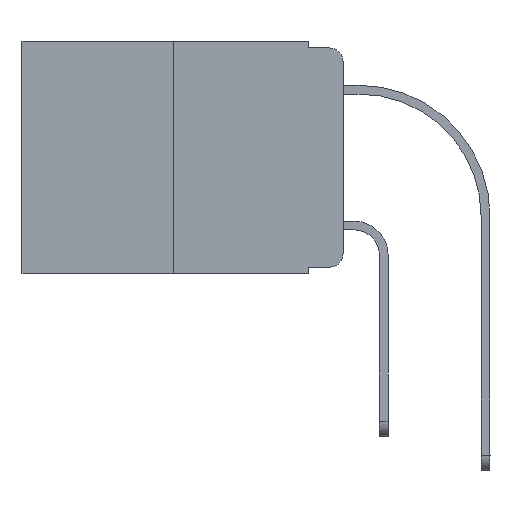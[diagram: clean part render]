
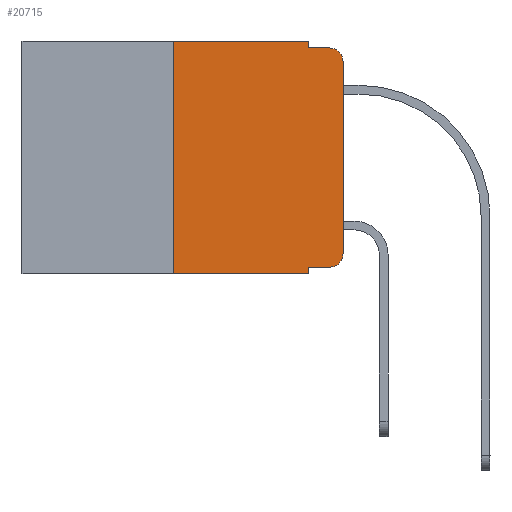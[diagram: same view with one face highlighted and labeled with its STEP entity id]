
A CAD part, left-side view. The second image highlights one B-rep face of the part: STEP entity #20715.
In plain terms, the highlighted planar face has unit normal (-1, 0, 0).
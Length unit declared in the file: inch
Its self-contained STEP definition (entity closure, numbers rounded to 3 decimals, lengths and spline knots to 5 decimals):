
#420 = DIRECTION ( 'NONE',  ( 0., 0., -1. ) ) ;
#704 = LINE ( 'NONE', #15815, #18201 ) ;
#1155 = CARTESIAN_POINT ( 'NONE',  ( 0., 0.051, -0.01 ) ) ;
#1318 = LINE ( 'NONE', #11101, #2013 ) ;
#1410 = EDGE_CURVE ( 'NONE', #24052, #24113, #2910, .T. ) ;
#1535 = DIRECTION ( 'NONE',  ( 0., -1., 0. ) ) ;
#2013 = VECTOR ( 'NONE', #20582, 39.37008 ) ;
#2109 = CARTESIAN_POINT ( 'NONE',  ( 0., 0.02, -0.01 ) ) ;
#2423 = EDGE_CURVE ( 'NONE', #16478, #14623, #15727, .T. ) ;
#2548 = ORIENTED_EDGE ( 'NONE', *, *, #1410, .F. ) ;
#2594 = LINE ( 'NONE', #12363, #2816 ) ;
#2816 = VECTOR ( 'NONE', #10336, 39.37008 ) ;
#2910 = LINE ( 'NONE', #12431, #20098 ) ;
#2971 = VERTEX_POINT ( 'NONE', #6167 ) ;
#3082 = ORIENTED_EDGE ( 'NONE', *, *, #23763, .T. ) ;
#3496 = VECTOR ( 'NONE', #12062, 39.37008 ) ;
#4196 = EDGE_CURVE ( 'NONE', #17796, #24052, #704, .T. ) ;
#4217 = LINE ( 'NONE', #7647, #15035 ) ;
#4219 = ORIENTED_EDGE ( 'NONE', *, *, #4196, .F. ) ;
#5891 = EDGE_CURVE ( 'NONE', #14530, #2971, #2594, .T. ) ;
#6167 = CARTESIAN_POINT ( 'NONE',  ( 0., 0., -0.03 ) ) ;
#7014 = CARTESIAN_POINT ( 'NONE',  ( 0., 0.473, 0. ) ) ;
#7241 = LINE ( 'NONE', #1155, #8109 ) ;
#7606 = ORIENTED_EDGE ( 'NONE', *, *, #24341, .T. ) ;
#7647 = CARTESIAN_POINT ( 'NONE',  ( 0., 0.051, 0. ) ) ;
#8109 = VECTOR ( 'NONE', #1535, 39.37008 ) ;
#8528 = CARTESIAN_POINT ( 'NONE',  ( 0., 0.051, 0. ) ) ;
#9140 = CARTESIAN_POINT ( 'NONE',  ( 0., 0.051, -0.01 ) ) ;
#9180 = DIRECTION ( 'NONE',  ( 0., 0., -1. ) ) ;
#9775 = VERTEX_POINT ( 'NONE', #9140 ) ;
#9787 = DIRECTION ( 'NONE',  ( 0., 0., -1. ) ) ;
#9946 = VECTOR ( 'NONE', #18331, 39.37008 ) ;
#10307 = VERTEX_POINT ( 'NONE', #2109 ) ;
#10336 = DIRECTION ( 'NONE',  ( 0., 0., 1. ) ) ;
#10537 = EDGE_CURVE ( 'NONE', #17796, #14623, #14666, .T. ) ;
#10985 = AXIS2_PLACEMENT_3D ( 'NONE', #15717, #17748, #9787 ) ;
#11101 = CARTESIAN_POINT ( 'NONE',  ( 0., 0.051, -0.333 ) ) ;
#11473 = DIRECTION ( 'NONE',  ( 0., 0., -1. ) ) ;
#11680 = VERTEX_POINT ( 'NONE', #16482 ) ;
#11714 = CARTESIAN_POINT ( 'NONE',  ( 0., 0., -0.313 ) ) ;
#11954 = CARTESIAN_POINT ( 'NONE',  ( 0., 0.051, -0.343 ) ) ;
#12062 = DIRECTION ( 'NONE',  ( 0., 0., -1. ) ) ;
#12363 = CARTESIAN_POINT ( 'NONE',  ( 0., 0., 0. ) ) ;
#12381 = CARTESIAN_POINT ( 'NONE',  ( 0., 0.473, -0.343 ) ) ;
#12431 = CARTESIAN_POINT ( 'NONE',  ( 0., 0.473, 0. ) ) ;
#13005 = DIRECTION ( 'NONE',  ( -1., 0., 0. ) ) ;
#13034 = ORIENTED_EDGE ( 'NONE', *, *, #2423, .F. ) ;
#13130 = DIRECTION ( 'NONE',  ( 1., 0., 0. ) ) ;
#14486 = CARTESIAN_POINT ( 'NONE',  ( 0., 0.25, 0. ) ) ;
#14530 = VERTEX_POINT ( 'NONE', #11714 ) ;
#14623 = VERTEX_POINT ( 'NONE', #11954 ) ;
#14660 = ORIENTED_EDGE ( 'NONE', *, *, #20762, .T. ) ;
#14666 = LINE ( 'NONE', #12381, #9946 ) ;
#15035 = VECTOR ( 'NONE', #420, 39.37008 ) ;
#15155 = ORIENTED_EDGE ( 'NONE', *, *, #5891, .T. ) ;
#15717 = CARTESIAN_POINT ( 'NONE',  ( 0., 0.02, -0.313 ) ) ;
#15727 = LINE ( 'NONE', #19402, #3496 ) ;
#15815 = CARTESIAN_POINT ( 'NONE',  ( 0., 0.25, 0. ) ) ;
#16184 = DIRECTION ( 'NONE',  ( 0., 0., 1. ) ) ;
#16301 = AXIS2_PLACEMENT_3D ( 'NONE', #22598, #13005, #9180 ) ;
#16460 = CARTESIAN_POINT ( 'NONE',  ( 0., 0.25, -0.343 ) ) ;
#16478 = VERTEX_POINT ( 'NONE', #20121 ) ;
#16482 = CARTESIAN_POINT ( 'NONE',  ( 0., 0.02, -0.333 ) ) ;
#17324 = ORIENTED_EDGE ( 'NONE', *, *, #10537, .T. ) ;
#17748 = DIRECTION ( 'NONE',  ( -1., 0., 0. ) ) ;
#17796 = VERTEX_POINT ( 'NONE', #16460 ) ;
#18201 = VECTOR ( 'NONE', #16184, 39.37008 ) ;
#18331 = DIRECTION ( 'NONE',  ( 0., -1., 0. ) ) ;
#18682 = FACE_OUTER_BOUND ( 'NONE', #19173, .T. ) ;
#19022 = EDGE_CURVE ( 'NONE', #24113, #9775, #4217, .T. ) ;
#19173 = EDGE_LOOP ( 'NONE', ( #15155, #14660, #23285, #22761, #2548, #4219, #17324, #13034, #3082, #7606 ) ) ;
#19402 = CARTESIAN_POINT ( 'NONE',  ( 0., 0.051, 0. ) ) ;
#19444 = CIRCLE ( 'NONE', #10985, 0.02 ) ;
#20098 = VECTOR ( 'NONE', #23825, 39.37008 ) ;
#20121 = CARTESIAN_POINT ( 'NONE',  ( 0., 0.051, -0.333 ) ) ;
#20582 = DIRECTION ( 'NONE',  ( 0., -1., 0. ) ) ;
#20715 = ADVANCED_FACE ( 'NONE', ( #18682 ), #22735, .F. ) ;
#20762 = EDGE_CURVE ( 'NONE', #2971, #10307, #24389, .T. ) ;
#22598 = CARTESIAN_POINT ( 'NONE',  ( 0., 0.02, -0.03 ) ) ;
#22735 = PLANE ( 'NONE',  #23578 ) ;
#22761 = ORIENTED_EDGE ( 'NONE', *, *, #19022, .F. ) ;
#23285 = ORIENTED_EDGE ( 'NONE', *, *, #24244, .F. ) ;
#23578 = AXIS2_PLACEMENT_3D ( 'NONE', #7014, #13130, #11473 ) ;
#23763 = EDGE_CURVE ( 'NONE', #16478, #11680, #1318, .T. ) ;
#23825 = DIRECTION ( 'NONE',  ( 0., -1., 0. ) ) ;
#24052 = VERTEX_POINT ( 'NONE', #14486 ) ;
#24113 = VERTEX_POINT ( 'NONE', #8528 ) ;
#24244 = EDGE_CURVE ( 'NONE', #9775, #10307, #7241, .T. ) ;
#24341 = EDGE_CURVE ( 'NONE', #11680, #14530, #19444, .T. ) ;
#24389 = CIRCLE ( 'NONE', #16301, 0.02 ) ;
